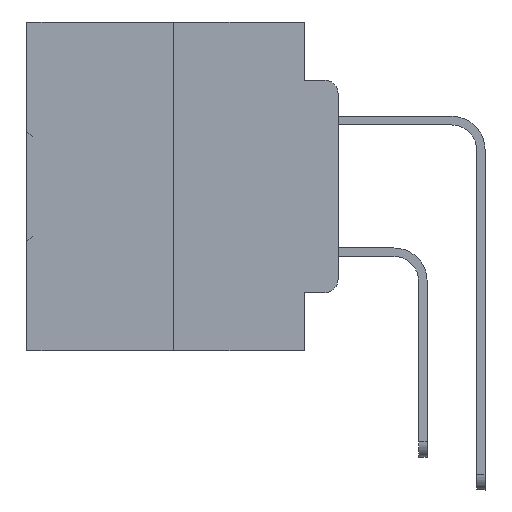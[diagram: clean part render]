
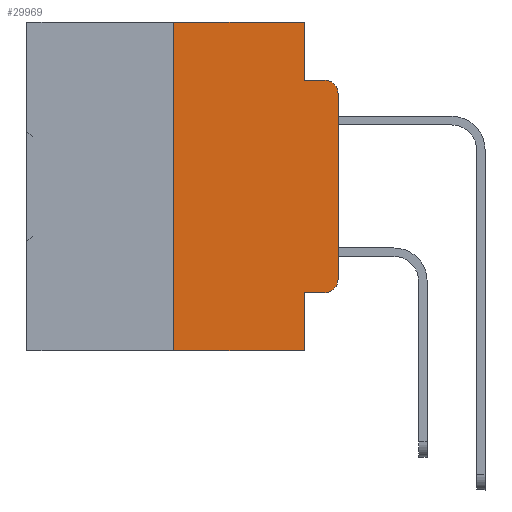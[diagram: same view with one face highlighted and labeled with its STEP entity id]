
A CAD part, left-side view. The second image highlights one B-rep face of the part: STEP entity #29969.
In plain terms, the highlighted planar face has unit normal (-1, 0, 0).
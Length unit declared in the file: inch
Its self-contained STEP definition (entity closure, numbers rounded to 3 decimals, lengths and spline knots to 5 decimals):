
#396 = DIRECTION ( 'NONE',  ( 0., 0., 1. ) ) ;
#554 = DIRECTION ( 'NONE',  ( 0., 0., -1. ) ) ;
#591 = EDGE_CURVE ( 'NONE', #30029, #17698, #5724, .T. ) ;
#858 = LINE ( 'NONE', #17305, #7222 ) ;
#867 = ORIENTED_EDGE ( 'NONE', *, *, #11037, .T. ) ;
#1020 = CARTESIAN_POINT ( 'NONE',  ( 0., 0.25, -0.5 ) ) ;
#2192 = CARTESIAN_POINT ( 'NONE',  ( 0., 0., -0.3915 ) ) ;
#2310 = EDGE_CURVE ( 'NONE', #7772, #17698, #31023, .T. ) ;
#2618 = CARTESIAN_POINT ( 'NONE',  ( 0., 0.02, -0.4115 ) ) ;
#3865 = DIRECTION ( 'NONE',  ( -1., 0., 0. ) ) ;
#5026 = AXIS2_PLACEMENT_3D ( 'NONE', #22722, #3865, #17355 ) ;
#5537 = ORIENTED_EDGE ( 'NONE', *, *, #16187, .F. ) ;
#5724 = LINE ( 'NONE', #17004, #33938 ) ;
#5726 = VERTEX_POINT ( 'NONE', #22879 ) ;
#5803 = LINE ( 'NONE', #20047, #26180 ) ;
#6054 = LINE ( 'NONE', #11819, #24497 ) ;
#6193 = EDGE_LOOP ( 'NONE', ( #12525, #867, #5537, #31891, #11839, #17295, #21659, #28157, #11743, #27294 ) ) ;
#6394 = CARTESIAN_POINT ( 'NONE',  ( 0., 0., -0.1085 ) ) ;
#7222 = VECTOR ( 'NONE', #12337, 39.37008 ) ;
#7772 = VERTEX_POINT ( 'NONE', #1020 ) ;
#7934 = CIRCLE ( 'NONE', #16216, 0.02 ) ;
#8120 = CARTESIAN_POINT ( 'NONE',  ( 0., 0.051, -0.5 ) ) ;
#8329 = VERTEX_POINT ( 'NONE', #15926 ) ;
#8772 = CARTESIAN_POINT ( 'NONE',  ( 0., 0.473, 0. ) ) ;
#9625 = CARTESIAN_POINT ( 'NONE',  ( 0., 0.25, 0. ) ) ;
#10001 = LINE ( 'NONE', #34924, #25878 ) ;
#10420 = VERTEX_POINT ( 'NONE', #6394 ) ;
#11037 = EDGE_CURVE ( 'NONE', #10420, #18453, #7934, .T. ) ;
#11743 = ORIENTED_EDGE ( 'NONE', *, *, #21746, .T. ) ;
#11819 = CARTESIAN_POINT ( 'NONE',  ( 0., 0.051, 0. ) ) ;
#11839 = ORIENTED_EDGE ( 'NONE', *, *, #36359, .F. ) ;
#12279 = CARTESIAN_POINT ( 'NONE',  ( 0., 0.02, -0.1085 ) ) ;
#12337 = DIRECTION ( 'NONE',  ( 0., -1., 0. ) ) ;
#12525 = ORIENTED_EDGE ( 'NONE', *, *, #35584, .T. ) ;
#13614 = VECTOR ( 'NONE', #17140, 39.37008 ) ;
#14143 = PLANE ( 'NONE',  #20676 ) ;
#14878 = VERTEX_POINT ( 'NONE', #29794 ) ;
#15926 = CARTESIAN_POINT ( 'NONE',  ( 0., 0.051, 0. ) ) ;
#16187 = EDGE_CURVE ( 'NONE', #14878, #18453, #10001, .T. ) ;
#16216 = AXIS2_PLACEMENT_3D ( 'NONE', #12279, #23886, #28215 ) ;
#17004 = CARTESIAN_POINT ( 'NONE',  ( 0., 0.051, 0. ) ) ;
#17140 = DIRECTION ( 'NONE',  ( 0., -1., 0. ) ) ;
#17295 = ORIENTED_EDGE ( 'NONE', *, *, #27444, .F. ) ;
#17305 = CARTESIAN_POINT ( 'NONE',  ( 0., 0.051, -0.4115 ) ) ;
#17355 = DIRECTION ( 'NONE',  ( 0., 0., -1. ) ) ;
#17698 = VERTEX_POINT ( 'NONE', #8120 ) ;
#17901 = CARTESIAN_POINT ( 'NONE',  ( 0., 0.473, 0. ) ) ;
#18453 = VERTEX_POINT ( 'NONE', #32453 ) ;
#19395 = VERTEX_POINT ( 'NONE', #2618 ) ;
#20047 = CARTESIAN_POINT ( 'NONE',  ( 0., 0., 0. ) ) ;
#20676 = AXIS2_PLACEMENT_3D ( 'NONE', #8772, #34630, #31322 ) ;
#21453 = VERTEX_POINT ( 'NONE', #2192 ) ;
#21659 = ORIENTED_EDGE ( 'NONE', *, *, #2310, .T. ) ;
#21746 = EDGE_CURVE ( 'NONE', #30029, #19395, #858, .T. ) ;
#22685 = CARTESIAN_POINT ( 'NONE',  ( 0., 0.473, -0.5 ) ) ;
#22722 = CARTESIAN_POINT ( 'NONE',  ( 0., 0.02, -0.3915 ) ) ;
#22879 = CARTESIAN_POINT ( 'NONE',  ( 0., 0.25, 0. ) ) ;
#23167 = DIRECTION ( 'NONE',  ( 0., 0., 1. ) ) ;
#23448 = LINE ( 'NONE', #17901, #35691 ) ;
#23886 = DIRECTION ( 'NONE',  ( -1., 0., 0. ) ) ;
#24497 = VECTOR ( 'NONE', #34323, 39.37008 ) ;
#25878 = VECTOR ( 'NONE', #27156, 39.37008 ) ;
#25917 = EDGE_CURVE ( 'NONE', #8329, #14878, #6054, .T. ) ;
#26180 = VECTOR ( 'NONE', #23167, 39.37008 ) ;
#27156 = DIRECTION ( 'NONE',  ( 0., -1., 0. ) ) ;
#27294 = ORIENTED_EDGE ( 'NONE', *, *, #36363, .T. ) ;
#27444 = EDGE_CURVE ( 'NONE', #7772, #5726, #28485, .T. ) ;
#28157 = ORIENTED_EDGE ( 'NONE', *, *, #591, .F. ) ;
#28215 = DIRECTION ( 'NONE',  ( 0., 0., -1. ) ) ;
#28485 = LINE ( 'NONE', #9625, #33423 ) ;
#29186 = DIRECTION ( 'NONE',  ( 0., -1., 0. ) ) ;
#29794 = CARTESIAN_POINT ( 'NONE',  ( 0., 0.051, -0.0885 ) ) ;
#29969 = ADVANCED_FACE ( 'NONE', ( #34073 ), #14143, .F. ) ;
#30029 = VERTEX_POINT ( 'NONE', #32598 ) ;
#31023 = LINE ( 'NONE', #22685, #13614 ) ;
#31322 = DIRECTION ( 'NONE',  ( 0., 0., -1. ) ) ;
#31891 = ORIENTED_EDGE ( 'NONE', *, *, #25917, .F. ) ;
#32453 = CARTESIAN_POINT ( 'NONE',  ( 0., 0.02, -0.0885 ) ) ;
#32598 = CARTESIAN_POINT ( 'NONE',  ( 0., 0.051, -0.4115 ) ) ;
#32750 = CIRCLE ( 'NONE', #5026, 0.02 ) ;
#33423 = VECTOR ( 'NONE', #396, 39.37008 ) ;
#33938 = VECTOR ( 'NONE', #554, 39.37008 ) ;
#34073 = FACE_OUTER_BOUND ( 'NONE', #6193, .T. ) ;
#34323 = DIRECTION ( 'NONE',  ( 0., 0., -1. ) ) ;
#34630 = DIRECTION ( 'NONE',  ( 1., 0., 0. ) ) ;
#34924 = CARTESIAN_POINT ( 'NONE',  ( 0., 0.051, -0.0885 ) ) ;
#35584 = EDGE_CURVE ( 'NONE', #21453, #10420, #5803, .T. ) ;
#35691 = VECTOR ( 'NONE', #29186, 39.37008 ) ;
#36359 = EDGE_CURVE ( 'NONE', #5726, #8329, #23448, .T. ) ;
#36363 = EDGE_CURVE ( 'NONE', #19395, #21453, #32750, .T. ) ;
